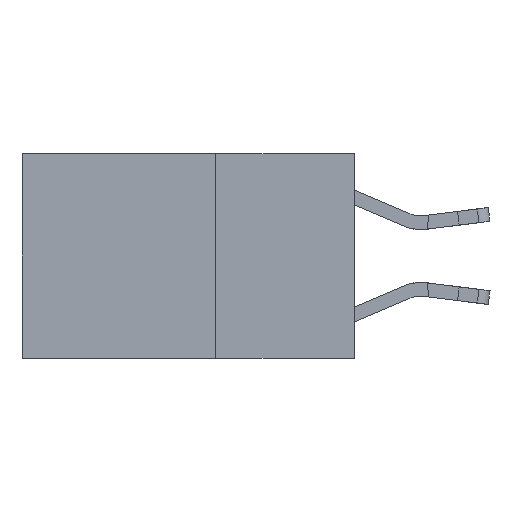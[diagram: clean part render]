
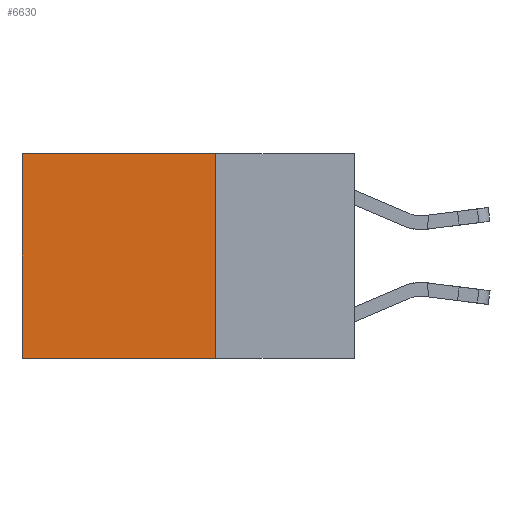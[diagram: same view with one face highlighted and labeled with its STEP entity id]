
A CAD part, left-side view. The second image highlights one B-rep face of the part: STEP entity #6630.
In plain terms, the highlighted planar face has unit normal (-1, 0, 0).
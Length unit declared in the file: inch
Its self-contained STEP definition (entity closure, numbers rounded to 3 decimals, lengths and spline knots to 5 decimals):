
#1023 = VECTOR ( 'NONE', #15889, 39.37008 ) ;
#1886 = PLANE ( 'NONE',  #12279 ) ;
#1966 = CARTESIAN_POINT ( 'NONE',  ( 0.2625, 0.25, 0. ) ) ;
#3327 = CARTESIAN_POINT ( 'NONE',  ( 0.2625, 0.25, 0. ) ) ;
#4382 = CARTESIAN_POINT ( 'NONE',  ( 0.2625, 0.6, 0. ) ) ;
#4416 = CARTESIAN_POINT ( 'NONE',  ( 0.2625, 0.25, -0.37 ) ) ;
#4513 = ORIENTED_EDGE ( 'NONE', *, *, #7651, .F. ) ;
#4768 = EDGE_CURVE ( 'NONE', #20382, #11046, #9599, .T. ) ;
#5121 = DIRECTION ( 'NONE',  ( 1., 0., 0. ) ) ;
#5671 = EDGE_LOOP ( 'NONE', ( #8303, #4513, #15660, #9269 ) ) ;
#5761 = LINE ( 'NONE', #4382, #14249 ) ;
#6057 = VERTEX_POINT ( 'NONE', #14196 ) ;
#6630 = ADVANCED_FACE ( 'NONE', ( #20189 ), #1886, .F. ) ;
#6870 = DIRECTION ( 'NONE',  ( 0., 1., 0. ) ) ;
#7651 = EDGE_CURVE ( 'NONE', #11046, #6057, #20177, .T. ) ;
#8275 = CARTESIAN_POINT ( 'NONE',  ( 0.2625, 0.6, 0. ) ) ;
#8303 = ORIENTED_EDGE ( 'NONE', *, *, #17984, .T. ) ;
#9250 = DIRECTION ( 'NONE',  ( 0., 0., -1. ) ) ;
#9269 = ORIENTED_EDGE ( 'NONE', *, *, #19263, .T. ) ;
#9599 = LINE ( 'NONE', #20657, #1023 ) ;
#10792 = CARTESIAN_POINT ( 'NONE',  ( 0.2625, 0.25, -0.37 ) ) ;
#11046 = VERTEX_POINT ( 'NONE', #4416 ) ;
#12279 = AXIS2_PLACEMENT_3D ( 'NONE', #14710, #5121, #16286 ) ;
#14196 = CARTESIAN_POINT ( 'NONE',  ( 0.2625, 0.6, -0.37 ) ) ;
#14249 = VECTOR ( 'NONE', #9250, 39.37008 ) ;
#14710 = CARTESIAN_POINT ( 'NONE',  ( 0.2625, 0.25, 0. ) ) ;
#14757 = VECTOR ( 'NONE', #6870, 39.37008 ) ;
#15250 = LINE ( 'NONE', #1966, #14757 ) ;
#15660 = ORIENTED_EDGE ( 'NONE', *, *, #4768, .F. ) ;
#15889 = DIRECTION ( 'NONE',  ( 0., 0., -1. ) ) ;
#16286 = DIRECTION ( 'NONE',  ( 0., 0., -1. ) ) ;
#16464 = VECTOR ( 'NONE', #20257, 39.37008 ) ;
#17984 = EDGE_CURVE ( 'NONE', #18477, #6057, #5761, .T. ) ;
#18477 = VERTEX_POINT ( 'NONE', #8275 ) ;
#19263 = EDGE_CURVE ( 'NONE', #20382, #18477, #15250, .T. ) ;
#20177 = LINE ( 'NONE', #10792, #16464 ) ;
#20189 = FACE_OUTER_BOUND ( 'NONE', #5671, .T. ) ;
#20257 = DIRECTION ( 'NONE',  ( 0., 1., 0. ) ) ;
#20382 = VERTEX_POINT ( 'NONE', #3327 ) ;
#20657 = CARTESIAN_POINT ( 'NONE',  ( 0.2625, 0.25, 0. ) ) ;
